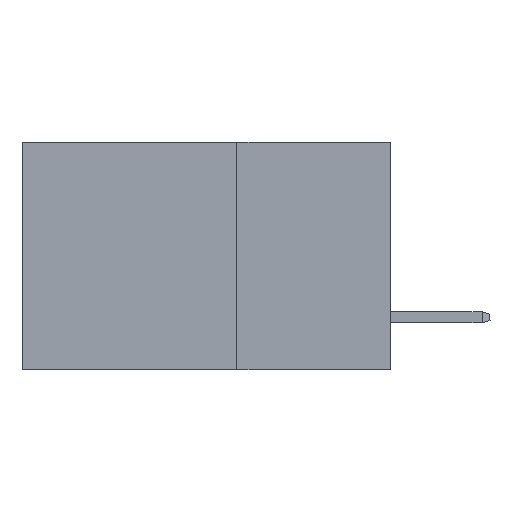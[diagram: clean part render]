
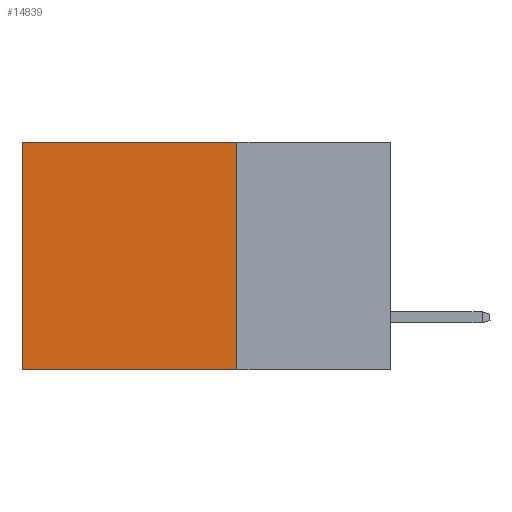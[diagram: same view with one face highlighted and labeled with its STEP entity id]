
A CAD part, left-side view. The second image highlights one B-rep face of the part: STEP entity #14839.
In plain terms, the highlighted planar face has unit normal (-1, 0, 0).
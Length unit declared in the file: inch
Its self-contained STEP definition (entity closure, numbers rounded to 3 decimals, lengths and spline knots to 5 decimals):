
#1042 = FACE_OUTER_BOUND ( 'NONE', #16216, .T. ) ;
#1492 = CARTESIAN_POINT ( 'NONE',  ( 0.2875, 0.6, 0. ) ) ;
#2689 = ORIENTED_EDGE ( 'NONE', *, *, #4775, .F. ) ;
#3207 = VECTOR ( 'NONE', #20383, 39.37008 ) ;
#3483 = VERTEX_POINT ( 'NONE', #23159 ) ;
#4523 = CARTESIAN_POINT ( 'NONE',  ( 0.2875, 0.25, 0. ) ) ;
#4775 = EDGE_CURVE ( 'NONE', #3483, #24655, #22039, .T. ) ;
#5089 = DIRECTION ( 'NONE',  ( 0., 0., -1. ) ) ;
#6088 = LINE ( 'NONE', #26265, #25798 ) ;
#7498 = PLANE ( 'NONE',  #12983 ) ;
#7514 = DIRECTION ( 'NONE',  ( 0., 1., 0. ) ) ;
#9439 = VERTEX_POINT ( 'NONE', #18187 ) ;
#9566 = LINE ( 'NONE', #1492, #3207 ) ;
#12906 = DIRECTION ( 'NONE',  ( 0., 0., -1. ) ) ;
#12983 = AXIS2_PLACEMENT_3D ( 'NONE', #20900, #28905, #12906 ) ;
#14671 = ORIENTED_EDGE ( 'NONE', *, *, #21393, .T. ) ;
#14839 = ADVANCED_FACE ( 'NONE', ( #1042 ), #7498, .F. ) ;
#15050 = ORIENTED_EDGE ( 'NONE', *, *, #33972, .T. ) ;
#16216 = EDGE_LOOP ( 'NONE', ( #14671, #30493, #2689, #15050 ) ) ;
#18187 = CARTESIAN_POINT ( 'NONE',  ( 0.2875, 0.6, -0.37 ) ) ;
#18743 = VECTOR ( 'NONE', #20649, 39.37008 ) ;
#20373 = CARTESIAN_POINT ( 'NONE',  ( 0.2875, 0.6, 0. ) ) ;
#20383 = DIRECTION ( 'NONE',  ( 0., 0., -1. ) ) ;
#20649 = DIRECTION ( 'NONE',  ( 0., 1., 0. ) ) ;
#20900 = CARTESIAN_POINT ( 'NONE',  ( 0.2875, 0.25, 0. ) ) ;
#21393 = EDGE_CURVE ( 'NONE', #23561, #9439, #9566, .T. ) ;
#22039 = LINE ( 'NONE', #29100, #28250 ) ;
#23159 = CARTESIAN_POINT ( 'NONE',  ( 0.2875, 0.25, 0. ) ) ;
#23561 = VERTEX_POINT ( 'NONE', #20373 ) ;
#24655 = VERTEX_POINT ( 'NONE', #33492 ) ;
#24976 = LINE ( 'NONE', #4523, #18743 ) ;
#25798 = VECTOR ( 'NONE', #7514, 39.37008 ) ;
#26265 = CARTESIAN_POINT ( 'NONE',  ( 0.2875, 0.25, -0.37 ) ) ;
#28250 = VECTOR ( 'NONE', #5089, 39.37008 ) ;
#28905 = DIRECTION ( 'NONE',  ( 1., 0., 0. ) ) ;
#29100 = CARTESIAN_POINT ( 'NONE',  ( 0.2875, 0.25, 0. ) ) ;
#30493 = ORIENTED_EDGE ( 'NONE', *, *, #33519, .F. ) ;
#33492 = CARTESIAN_POINT ( 'NONE',  ( 0.2875, 0.25, -0.37 ) ) ;
#33519 = EDGE_CURVE ( 'NONE', #24655, #9439, #6088, .T. ) ;
#33972 = EDGE_CURVE ( 'NONE', #3483, #23561, #24976, .T. ) ;
